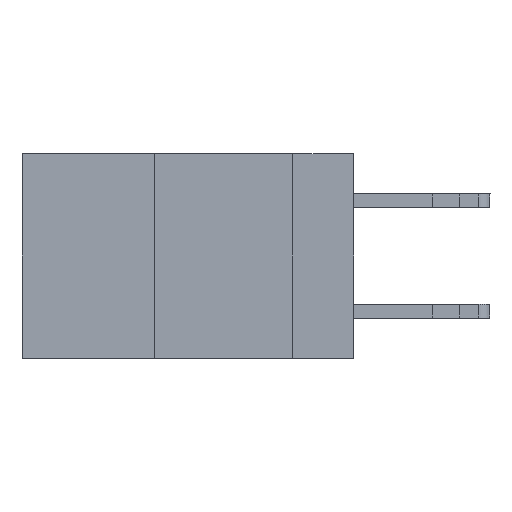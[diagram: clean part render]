
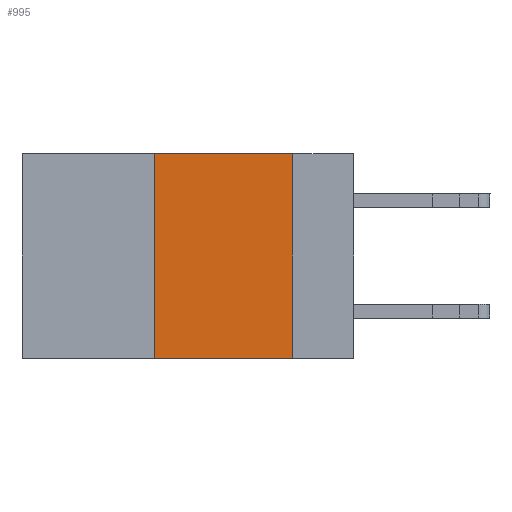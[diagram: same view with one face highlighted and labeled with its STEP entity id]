
A CAD part, left-side view. The second image highlights one B-rep face of the part: STEP entity #995.
In plain terms, the highlighted planar face has unit normal (-1, 0, 0).
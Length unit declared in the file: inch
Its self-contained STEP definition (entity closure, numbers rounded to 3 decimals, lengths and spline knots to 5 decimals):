
#640 = DIRECTION ( 'NONE',  ( 0., 0., -1. ) ) ;
#995 = ADVANCED_FACE ( 'NONE', ( #2579 ), #12106, .F. ) ;
#1175 = CARTESIAN_POINT ( 'NONE',  ( 0., 0.36, -0.37 ) ) ;
#1930 = LINE ( 'NONE', #19770, #10129 ) ;
#2188 = ORIENTED_EDGE ( 'NONE', *, *, #13679, .F. ) ;
#2365 = LINE ( 'NONE', #20075, #20947 ) ;
#2389 = EDGE_CURVE ( 'NONE', #2484, #11118, #2365, .T. ) ;
#2484 = VERTEX_POINT ( 'NONE', #1175 ) ;
#2579 = FACE_OUTER_BOUND ( 'NONE', #4981, .T. ) ;
#2942 = LINE ( 'NONE', #15891, #12022 ) ;
#4981 = EDGE_LOOP ( 'NONE', ( #2188, #6084, #9889, #7844 ) ) ;
#5083 = DIRECTION ( 'NONE',  ( 0., 0., 1. ) ) ;
#5229 = AXIS2_PLACEMENT_3D ( 'NONE', #10509, #17228, #640 ) ;
#5796 = CARTESIAN_POINT ( 'NONE',  ( 0., 0.11, 0. ) ) ;
#6084 = ORIENTED_EDGE ( 'NONE', *, *, #17943, .F. ) ;
#6972 = CARTESIAN_POINT ( 'NONE',  ( 0., 0.11, -0.37 ) ) ;
#7367 = VERTEX_POINT ( 'NONE', #5796 ) ;
#7632 = VECTOR ( 'NONE', #5083, 39.37008 ) ;
#7844 = ORIENTED_EDGE ( 'NONE', *, *, #2389, .T. ) ;
#9705 = LINE ( 'NONE', #13010, #7632 ) ;
#9889 = ORIENTED_EDGE ( 'NONE', *, *, #15061, .F. ) ;
#10129 = VECTOR ( 'NONE', #11595, 39.37008 ) ;
#10509 = CARTESIAN_POINT ( 'NONE',  ( 0., 0.6, 0. ) ) ;
#11118 = VERTEX_POINT ( 'NONE', #6972 ) ;
#11595 = DIRECTION ( 'NONE',  ( 0., -1., 0. ) ) ;
#12022 = VECTOR ( 'NONE', #17273, 39.37008 ) ;
#12106 = PLANE ( 'NONE',  #5229 ) ;
#13010 = CARTESIAN_POINT ( 'NONE',  ( 0., 0.36, 0. ) ) ;
#13332 = CARTESIAN_POINT ( 'NONE',  ( 0., 0.36, 0. ) ) ;
#13679 = EDGE_CURVE ( 'NONE', #7367, #11118, #2942, .T. ) ;
#15061 = EDGE_CURVE ( 'NONE', #2484, #17532, #9705, .T. ) ;
#15312 = DIRECTION ( 'NONE',  ( 0., -1., 0. ) ) ;
#15891 = CARTESIAN_POINT ( 'NONE',  ( 0., 0.11, 0. ) ) ;
#17228 = DIRECTION ( 'NONE',  ( 1., 0., 0. ) ) ;
#17273 = DIRECTION ( 'NONE',  ( 0., 0., -1. ) ) ;
#17532 = VERTEX_POINT ( 'NONE', #13332 ) ;
#17943 = EDGE_CURVE ( 'NONE', #17532, #7367, #1930, .T. ) ;
#19770 = CARTESIAN_POINT ( 'NONE',  ( 0., 0.6, 0. ) ) ;
#20075 = CARTESIAN_POINT ( 'NONE',  ( 0., 0.6, -0.37 ) ) ;
#20947 = VECTOR ( 'NONE', #15312, 39.37008 ) ;
